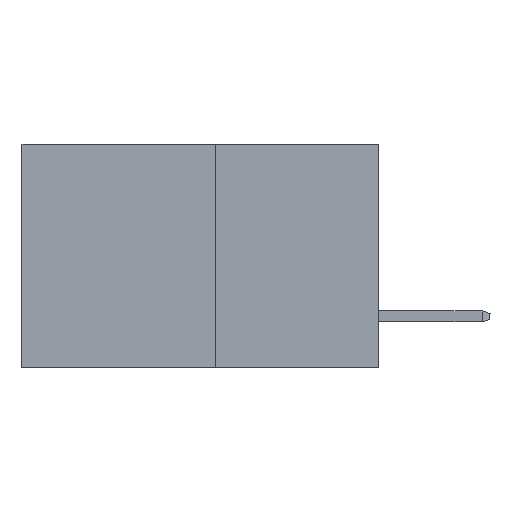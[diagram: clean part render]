
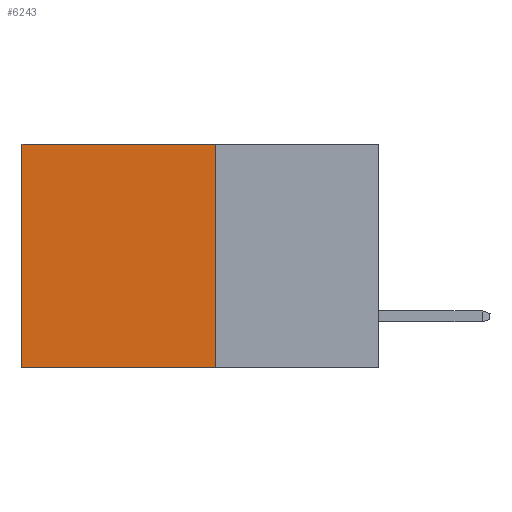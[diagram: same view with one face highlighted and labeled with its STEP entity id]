
A CAD part, left-side view. The second image highlights one B-rep face of the part: STEP entity #6243.
In plain terms, the highlighted planar face has unit normal (-1, 0, 0).
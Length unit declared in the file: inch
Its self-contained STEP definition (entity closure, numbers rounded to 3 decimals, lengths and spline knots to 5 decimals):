
#45 = EDGE_CURVE ( 'NONE', #4887, #5635, #4518, .T. ) ;
#1621 = DIRECTION ( 'NONE',  ( 0., 0., -1. ) ) ;
#1812 = ORIENTED_EDGE ( 'NONE', *, *, #2405, .T. ) ;
#1936 = DIRECTION ( 'NONE',  ( 0., 1., 0. ) ) ;
#1941 = EDGE_CURVE ( 'NONE', #7683, #5411, #11749, .T. ) ;
#2101 = DIRECTION ( 'NONE',  ( 0., 1., 0. ) ) ;
#2251 = ORIENTED_EDGE ( 'NONE', *, *, #1941, .F. ) ;
#2405 = EDGE_CURVE ( 'NONE', #5635, #5411, #3471, .T. ) ;
#2892 = DIRECTION ( 'NONE',  ( 0., 0., -1. ) ) ;
#3211 = VECTOR ( 'NONE', #2892, 39.37008 ) ;
#3471 = LINE ( 'NONE', #5983, #10411 ) ;
#3681 = EDGE_LOOP ( 'NONE', ( #1812, #2251, #4021, #4513 ) ) ;
#3765 = CARTESIAN_POINT ( 'NONE',  ( 0.277, 0.27, 0. ) ) ;
#3880 = VECTOR ( 'NONE', #2101, 39.37008 ) ;
#4021 = ORIENTED_EDGE ( 'NONE', *, *, #5573, .F. ) ;
#4513 = ORIENTED_EDGE ( 'NONE', *, *, #45, .T. ) ;
#4518 = LINE ( 'NONE', #6943, #3880 ) ;
#4887 = VERTEX_POINT ( 'NONE', #3765 ) ;
#4903 = FACE_OUTER_BOUND ( 'NONE', #3681, .T. ) ;
#5411 = VERTEX_POINT ( 'NONE', #5626 ) ;
#5573 = EDGE_CURVE ( 'NONE', #4887, #7683, #8187, .T. ) ;
#5626 = CARTESIAN_POINT ( 'NONE',  ( 0.277, 0.59, -0.37 ) ) ;
#5635 = VERTEX_POINT ( 'NONE', #8552 ) ;
#5658 = CARTESIAN_POINT ( 'NONE',  ( 0.277, 0.27, -0.37 ) ) ;
#5983 = CARTESIAN_POINT ( 'NONE',  ( 0.277, 0.59, -0.37 ) ) ;
#6178 = DIRECTION ( 'NONE',  ( 0., 0., -1. ) ) ;
#6243 = ADVANCED_FACE ( 'NONE', ( #4903 ), #6556, .F. ) ;
#6556 = PLANE ( 'NONE',  #8248 ) ;
#6943 = CARTESIAN_POINT ( 'NONE',  ( 0.277, 0.27, 0. ) ) ;
#7447 = DIRECTION ( 'NONE',  ( 1., 0., 0. ) ) ;
#7618 = CARTESIAN_POINT ( 'NONE',  ( 0.277, 0.27, -0.37 ) ) ;
#7683 = VERTEX_POINT ( 'NONE', #9860 ) ;
#8187 = LINE ( 'NONE', #7618, #3211 ) ;
#8248 = AXIS2_PLACEMENT_3D ( 'NONE', #5658, #7447, #1621 ) ;
#8478 = CARTESIAN_POINT ( 'NONE',  ( 0.277, 0.27, -0.37 ) ) ;
#8552 = CARTESIAN_POINT ( 'NONE',  ( 0.277, 0.59, 0. ) ) ;
#9237 = VECTOR ( 'NONE', #1936, 39.37008 ) ;
#9860 = CARTESIAN_POINT ( 'NONE',  ( 0.277, 0.27, -0.37 ) ) ;
#10411 = VECTOR ( 'NONE', #6178, 39.37008 ) ;
#11749 = LINE ( 'NONE', #8478, #9237 ) ;
